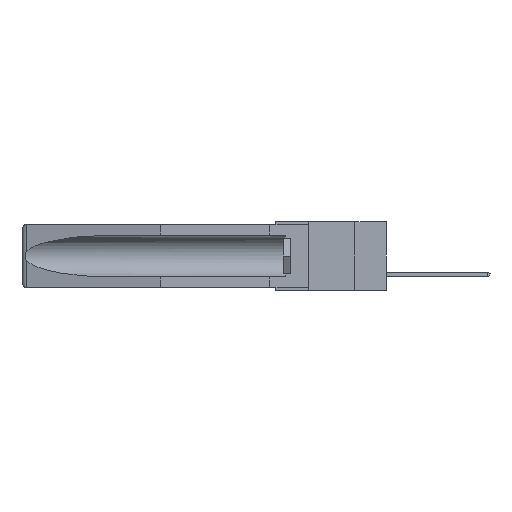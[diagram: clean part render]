
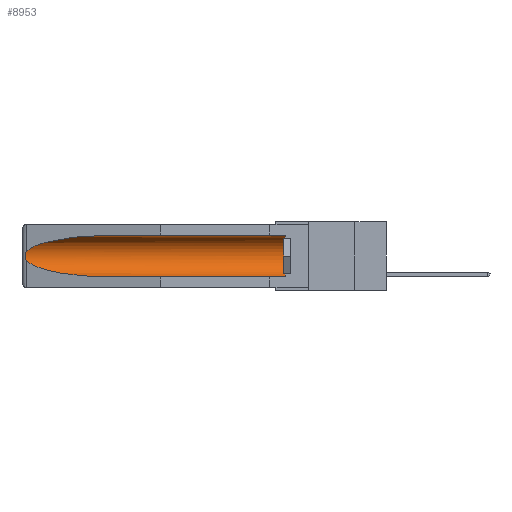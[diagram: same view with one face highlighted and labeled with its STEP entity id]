
A CAD part, left-side view. The second image highlights one B-rep face of the part: STEP entity #8953.
In plain terms, the highlighted cylindrical face has radius 2.857 mm (diameter 5.715 mm), a partial arc.
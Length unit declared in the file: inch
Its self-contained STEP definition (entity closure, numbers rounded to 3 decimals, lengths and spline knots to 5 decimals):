
#945 = LINE ( 'NONE', #4060, #14942 ) ;
#1396 = FACE_OUTER_BOUND ( 'NONE', #17211, .T. ) ;
#1972 = CARTESIAN_POINT ( 'NONE',  ( 0.26537, 1.52718, -0.19328 ) ) ;
#2053 = DIRECTION ( 'NONE',  ( 0., 1., 0. ) ) ;
#2867 = CARTESIAN_POINT ( 'NONE',  ( 0.26597, 1.52961, -0.15275 ) ) ;
#3332 = VERTEX_POINT ( 'NONE', #18611 ) ;
#3578 =( BOUNDED_CURVE ( )  B_SPLINE_CURVE ( 3, ( #15136, #11748, #16681, #13433 ),
 .UNSPECIFIED., .F., .F. ) 
 B_SPLINE_CURVE_WITH_KNOTS ( ( 4, 4 ),
 ( 4.71239, 6.08839 ),
 .UNSPECIFIED. ) 
 CURVE ( )  GEOMETRIC_REPRESENTATION_ITEM ( )  RATIONAL_B_SPLINE_CURVE ( ( 1., 0.848, 0.848, 1. ) ) 
 REPRESENTATION_ITEM ( '' )  );
#4060 = CARTESIAN_POINT ( 'NONE',  ( 0.155, -0.30754, -0.059 ) ) ;
#4195 = VERTEX_POINT ( 'NONE', #18509 ) ;
#4240 = ORIENTED_EDGE ( 'NONE', *, *, #10429, .T. ) ;
#4513 = CARTESIAN_POINT ( 'NONE',  ( 0.26537, 1.52718, -0.19328 ) ) ;
#4678 = ORIENTED_EDGE ( 'NONE', *, *, #5718, .T. ) ;
#4698 = CARTESIAN_POINT ( 'NONE',  ( 0.25451, 1.48313, -0.24835 ) ) ;
#5718 = EDGE_CURVE ( 'NONE', #4195, #8920, #20177, .T. ) ;
#5776 = VERTEX_POINT ( 'NONE', #9649 ) ;
#5826 = VERTEX_POINT ( 'NONE', #16730 ) ;
#6047 = ORIENTED_EDGE ( 'NONE', *, *, #18652, .T. ) ;
#6504 = CARTESIAN_POINT ( 'NONE',  ( 0.155, 0.126, -0.059 ) ) ;
#6564 = CARTESIAN_POINT ( 'NONE',  ( 0.155, 0.126, -0.1715 ) ) ;
#7470 = CARTESIAN_POINT ( 'NONE',  ( 0.26537, 1.52718, -0.14972 ) ) ;
#7617 = CARTESIAN_POINT ( 'NONE',  ( 0.2675, 1.53308, -0.16763 ) ) ;
#7721 = ORIENTED_EDGE ( 'NONE', *, *, #16029, .T. ) ;
#7752 = VECTOR ( 'NONE', #2053, 39.37008 ) ;
#7953 = CARTESIAN_POINT ( 'NONE',  ( 0.2673, 1.5327, -0.16383 ) ) ;
#8385 = ORIENTED_EDGE ( 'NONE', *, *, #8503, .T. ) ;
#8503 = EDGE_CURVE ( 'NONE', #5776, #8542, #18585, .T. ) ;
#8542 = VERTEX_POINT ( 'NONE', #6504 ) ;
#8672 = AXIS2_PLACEMENT_3D ( 'NONE', #6564, #15989, #17510 ) ;
#8920 = VERTEX_POINT ( 'NONE', #10726 ) ;
#8953 = ADVANCED_FACE ( 'NONE', ( #1396 ), #9989, .F. ) ;
#9649 = CARTESIAN_POINT ( 'NONE',  ( 0.155, 0.126, -0.284 ) ) ;
#9989 = CYLINDRICAL_SURFACE ( 'NONE', #16111, 0.1125 ) ;
#10148 = EDGE_CURVE ( 'NONE', #5776, #3332, #15329, .T. ) ;
#10327 = CARTESIAN_POINT ( 'NONE',  ( 0.26655, 1.53094, -0.18657 ) ) ;
#10429 = EDGE_CURVE ( 'NONE', #8920, #3332, #13548, .T. ) ;
#10726 = CARTESIAN_POINT ( 'NONE',  ( 0.26537, 1.52718, -0.19328 ) ) ;
#10883 = CARTESIAN_POINT ( 'NONE',  ( 0.155, -0.30754, -0.1715 ) ) ;
#11426 = CARTESIAN_POINT ( 'NONE',  ( 0.2673, 1.53269, -0.17917 ) ) ;
#11469 = CARTESIAN_POINT ( 'NONE',  ( 0.21114, 1.30732, -0.284 ) ) ;
#11748 = CARTESIAN_POINT ( 'NONE',  ( 0.21114, 1.30732, -0.059 ) ) ;
#12634 = DIRECTION ( 'NONE',  ( 0., 1., 0. ) ) ;
#13221 = DIRECTION ( 'NONE',  ( 0., 1., 0. ) ) ;
#13316 = CARTESIAN_POINT ( 'NONE',  ( 0.155, -0.30754, -0.284 ) ) ;
#13433 = CARTESIAN_POINT ( 'NONE',  ( 0.26537, 1.52718, -0.14972 ) ) ;
#13548 =( BOUNDED_CURVE ( )  B_SPLINE_CURVE ( 3, ( #1972, #4698, #11469, #15665 ),
 .UNSPECIFIED., .F., .F. ) 
 B_SPLINE_CURVE_WITH_KNOTS ( ( 4, 4 ),
 ( 0.1948, 1.5708 ),
 .UNSPECIFIED. ) 
 CURVE ( )  GEOMETRIC_REPRESENTATION_ITEM ( )  RATIONAL_B_SPLINE_CURVE ( ( 1., 0.848, 0.848, 1. ) ) 
 REPRESENTATION_ITEM ( '' )  );
#13662 = CARTESIAN_POINT ( 'NONE',  ( 0.2675, 1.53308, -0.17534 ) ) ;
#14942 = VECTOR ( 'NONE', #13221, 39.37008 ) ;
#15136 = CARTESIAN_POINT ( 'NONE',  ( 0.155, 1.07973, -0.059 ) ) ;
#15329 = LINE ( 'NONE', #13316, #7752 ) ;
#15419 = CARTESIAN_POINT ( 'NONE',  ( 0.26654, 1.53092, -0.15636 ) ) ;
#15665 = CARTESIAN_POINT ( 'NONE',  ( 0.155, 1.07973, -0.284 ) ) ;
#15989 = DIRECTION ( 'NONE',  ( 0., -1., 0. ) ) ;
#16029 = EDGE_CURVE ( 'NONE', #8542, #5826, #945, .T. ) ;
#16111 = AXIS2_PLACEMENT_3D ( 'NONE', #10883, #12634, #16992 ) ;
#16635 = ORIENTED_EDGE ( 'NONE', *, *, #10148, .F. ) ;
#16681 = CARTESIAN_POINT ( 'NONE',  ( 0.25451, 1.48313, -0.09465 ) ) ;
#16730 = CARTESIAN_POINT ( 'NONE',  ( 0.155, 1.07973, -0.059 ) ) ;
#16992 = DIRECTION ( 'NONE',  ( 0., 0., 1. ) ) ;
#17211 = EDGE_LOOP ( 'NONE', ( #6047, #4678, #4240, #16635, #8385, #7721 ) ) ;
#17510 = DIRECTION ( 'NONE',  ( 0., 0., 1. ) ) ;
#18509 = CARTESIAN_POINT ( 'NONE',  ( 0.26537, 1.52718, -0.14972 ) ) ;
#18585 = CIRCLE ( 'NONE', #8672, 0.1125 ) ;
#18611 = CARTESIAN_POINT ( 'NONE',  ( 0.155, 1.07973, -0.284 ) ) ;
#18652 = EDGE_CURVE ( 'NONE', #5826, #4195, #3578, .T. ) ;
#19142 = CARTESIAN_POINT ( 'NONE',  ( 0.26597, 1.5296, -0.19026 ) ) ;
#20177 = B_SPLINE_CURVE_WITH_KNOTS ( 'NONE', 3,
 ( #7470, #2867, #15419, #7953, #7617, #13662, #11426, #10327, #19142, #4513 ),
 .UNSPECIFIED., .F., .F.,
 ( 4, 2, 2, 2, 4 ),
 ( 0., 0.00029, 0.00058, 0.00087, 0.00117 ),
 .UNSPECIFIED. ) ;
